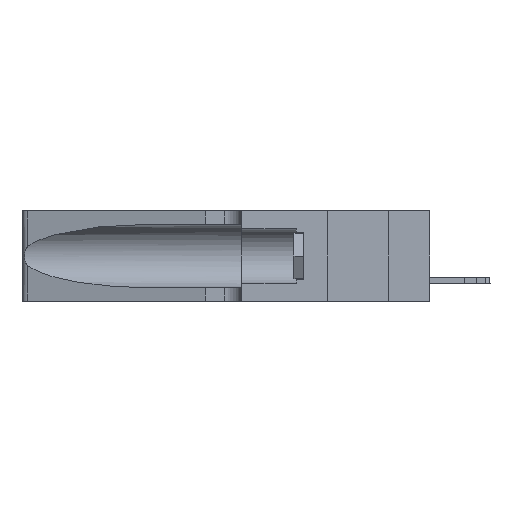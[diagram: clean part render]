
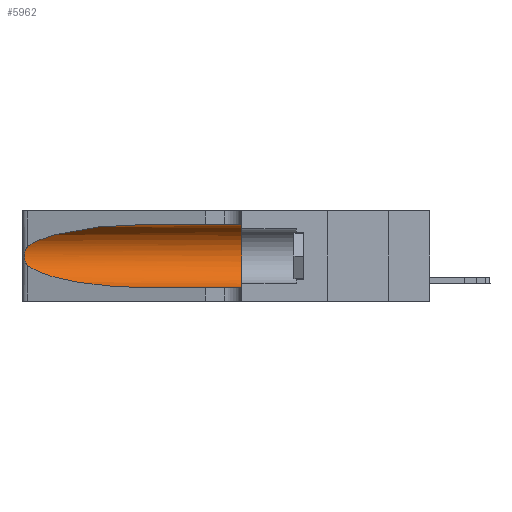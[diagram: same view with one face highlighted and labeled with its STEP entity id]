
A CAD part, left-side view. The second image highlights one B-rep face of the part: STEP entity #5962.
In plain terms, the highlighted cylindrical face has radius 3.308 mm (diameter 6.617 mm), a partial arc.
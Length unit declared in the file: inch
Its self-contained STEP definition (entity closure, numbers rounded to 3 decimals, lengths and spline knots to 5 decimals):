
#401 = CARTESIAN_POINT ( 'NONE',  ( 0.1305, 0.72297, 0.05475 ) ) ;
#586 = CARTESIAN_POINT ( 'NONE',  ( 0.1305, 0.35, 0.05475 ) ) ;
#1110 = CARTESIAN_POINT ( 'NONE',  ( 0.25787, 1.23484, 0.2124 ) ) ;
#1161 = LINE ( 'NONE', #11805, #4650 ) ;
#1201 = CARTESIAN_POINT ( 'NONE',  ( 0.26075, 1.23896, 0.19203 ) ) ;
#1457 = VERTEX_POINT ( 'NONE', #586 ) ;
#2767 = EDGE_CURVE ( 'NONE', #16766, #1457, #18394, .T. ) ;
#2985 = DIRECTION ( 'NONE',  ( 0., -1., 0. ) ) ;
#3305 = CARTESIAN_POINT ( 'NONE',  ( 0.18966, 0.96281, 0.05475 ) ) ;
#3337 = CARTESIAN_POINT ( 'NONE',  ( 0.26075, 1.23896, 0.178 ) ) ;
#3465 = VERTEX_POINT ( 'NONE', #18902 ) ;
#4226 = CYLINDRICAL_SURFACE ( 'NONE', #17045, 0.13025 ) ;
#4650 = VECTOR ( 'NONE', #18146, 39.37008 ) ;
#5375 = CARTESIAN_POINT ( 'NONE',  ( 0.25487, 1.22718, 0.22369 ) ) ;
#5962 = ADVANCED_FACE ( 'NONE', ( #10573 ), #4226, .F. ) ;
#6445 = EDGE_CURVE ( 'NONE', #3465, #10869, #26354, .T. ) ;
#6544 = CARTESIAN_POINT ( 'NONE',  ( 0.1305, 0.72297, 0.31525 ) ) ;
#7347 = CARTESIAN_POINT ( 'NONE',  ( 0.25856, 1.23593, 0.16098 ) ) ;
#7418 = CARTESIAN_POINT ( 'NONE',  ( 0.1305, 0.35, 0.185 ) ) ;
#7520 = CARTESIAN_POINT ( 'NONE',  ( 0.1305, 0.35, 0.31525 ) ) ;
#7529 = CARTESIAN_POINT ( 'NONE',  ( 0.25555, 1.22994, 0.2215 ) ) ;
#9238 = LINE ( 'NONE', #20628, #25842 ) ;
#9288 = CARTESIAN_POINT ( 'NONE',  ( 0.25639, 1.23184, 0.21858 ) ) ;
#9380 = CARTESIAN_POINT ( 'NONE',  ( 0.25789, 1.23486, 0.15765 ) ) ;
#9545 = CARTESIAN_POINT ( 'NONE',  ( 0.25639, 1.23186, 0.15144 ) ) ;
#10573 = FACE_OUTER_BOUND ( 'NONE', #13619, .T. ) ;
#10815 = VERTEX_POINT ( 'NONE', #19509 ) ;
#10869 = VERTEX_POINT ( 'NONE', #401 ) ;
#11105 = CARTESIAN_POINT ( 'NONE',  ( 0.25487, 1.22718, 0.14631 ) ) ;
#11110 = VERTEX_POINT ( 'NONE', #6544 ) ;
#11477 = DIRECTION ( 'NONE',  ( 0., 1., 0. ) ) ;
#11805 = CARTESIAN_POINT ( 'NONE',  ( 0.1305, 1.61858, 0.05475 ) ) ;
#12484 = CARTESIAN_POINT ( 'NONE',  ( 0.18966, 0.96281, 0.31525 ) ) ;
#12910 = ORIENTED_EDGE ( 'NONE', *, *, #17526, .T. ) ;
#13081 = ORIENTED_EDGE ( 'NONE', *, *, #23979, .F. ) ;
#13365 = CARTESIAN_POINT ( 'NONE',  ( 0.26018, 1.23835, 0.19895 ) ) ;
#13519 = DIRECTION ( 'NONE',  ( 0., 0., 1. ) ) ;
#13619 = EDGE_LOOP ( 'NONE', ( #14853, #12910, #21486, #22450, #22632, #13081 ) ) ;
#13844 = AXIS2_PLACEMENT_3D ( 'NONE', #7418, #11477, #13519 ) ;
#14853 = ORIENTED_EDGE ( 'NONE', *, *, #18519, .T. ) ;
#15351 = CARTESIAN_POINT ( 'NONE',  ( 0.25854, 1.2359, 0.20912 ) ) ;
#16680 = CARTESIAN_POINT ( 'NONE',  ( 0.2373, 1.15595, 0.28018 ) ) ;
#16766 = VERTEX_POINT ( 'NONE', #7520 ) ;
#17045 = AXIS2_PLACEMENT_3D ( 'NONE', #21042, #2985, #18918 ) ;
#17526 = EDGE_CURVE ( 'NONE', #10815, #3465, #24466, .T. ) ;
#18146 = DIRECTION ( 'NONE',  ( 0., -1., 0. ) ) ;
#18394 = CIRCLE ( 'NONE', #13844, 0.13025 ) ;
#18519 = EDGE_CURVE ( 'NONE', #11110, #10815, #20991, .T. ) ;
#18552 = CARTESIAN_POINT ( 'NONE',  ( 0.1305, 0.72297, 0.31525 ) ) ;
#18735 = CARTESIAN_POINT ( 'NONE',  ( 0.25487, 1.22718, 0.22369 ) ) ;
#18902 = CARTESIAN_POINT ( 'NONE',  ( 0.25487, 1.22718, 0.14631 ) ) ;
#18918 = DIRECTION ( 'NONE',  ( 0., 0., -1. ) ) ;
#19509 = CARTESIAN_POINT ( 'NONE',  ( 0.25487, 1.22718, 0.22369 ) ) ;
#19544 = CARTESIAN_POINT ( 'NONE',  ( 0.26017, 1.23833, 0.17102 ) ) ;
#19631 = CARTESIAN_POINT ( 'NONE',  ( 0.25555, 1.22993, 0.14849 ) ) ;
#20547 = DIRECTION ( 'NONE',  ( 0., -1., 0. ) ) ;
#20628 = CARTESIAN_POINT ( 'NONE',  ( 0.1305, 1.61858, 0.31525 ) ) ;
#20643 = EDGE_CURVE ( 'NONE', #10869, #1457, #1161, .T. ) ;
#20991 =( BOUNDED_CURVE ( )  B_SPLINE_CURVE ( 3, ( #18552, #12484, #16680, #18735 ),
 .UNSPECIFIED., .F., .T. ) 
 B_SPLINE_CURVE_WITH_KNOTS ( ( 4, 4 ),
 ( 1.5708, 2.84003 ),
 .UNSPECIFIED. ) 
 CURVE ( )  GEOMETRIC_REPRESENTATION_ITEM ( )  RATIONAL_B_SPLINE_CURVE ( ( 1., 0.87, 0.87, 1. ) ) 
 REPRESENTATION_ITEM ( '' )  );
#21042 = CARTESIAN_POINT ( 'NONE',  ( 0.1305, 1.61858, 0.185 ) ) ;
#21194 = CARTESIAN_POINT ( 'NONE',  ( 0.2373, 1.15595, 0.08982 ) ) ;
#21486 = ORIENTED_EDGE ( 'NONE', *, *, #6445, .T. ) ;
#22450 = ORIENTED_EDGE ( 'NONE', *, *, #20643, .T. ) ;
#22632 = ORIENTED_EDGE ( 'NONE', *, *, #2767, .F. ) ;
#23639 = CARTESIAN_POINT ( 'NONE',  ( 0.25487, 1.22718, 0.14631 ) ) ;
#23979 = EDGE_CURVE ( 'NONE', #11110, #16766, #9238, .T. ) ;
#24466 = B_SPLINE_CURVE_WITH_KNOTS ( 'NONE', 3,
 ( #5375, #7529, #9288, #1110, #15351, #13365, #1201, #3337, #19544, #7347, #9380, #9545, #19631, #23639 ),
 .UNSPECIFIED., .F., .F.,
 ( 4, 2, 2, 2, 2, 2, 4 ),
 ( 0., 0.00027, 0.00053, 0.00107, 0.0016, 0.00187, 0.00214 ),
 .UNSPECIFIED. ) ;
#25579 = CARTESIAN_POINT ( 'NONE',  ( 0.1305, 0.72297, 0.05475 ) ) ;
#25842 = VECTOR ( 'NONE', #20547, 39.37008 ) ;
#26354 =( BOUNDED_CURVE ( )  B_SPLINE_CURVE ( 3, ( #11105, #21194, #3305, #25579 ),
 .UNSPECIFIED., .F., .F. ) 
 B_SPLINE_CURVE_WITH_KNOTS ( ( 4, 4 ),
 ( 3.44316, 4.71239 ),
 .UNSPECIFIED. ) 
 CURVE ( )  GEOMETRIC_REPRESENTATION_ITEM ( )  RATIONAL_B_SPLINE_CURVE ( ( 1., 0.87, 0.87, 1. ) ) 
 REPRESENTATION_ITEM ( '' )  );
